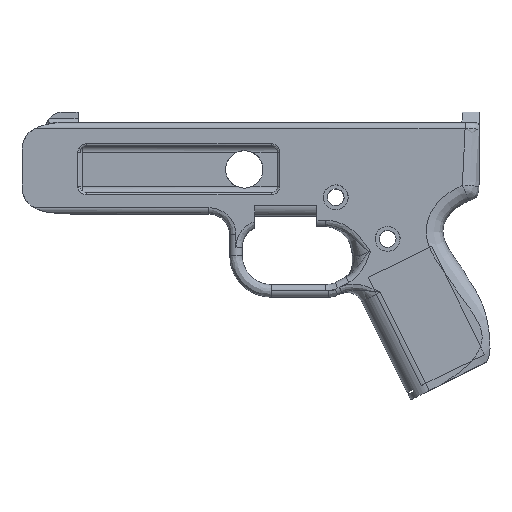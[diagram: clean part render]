
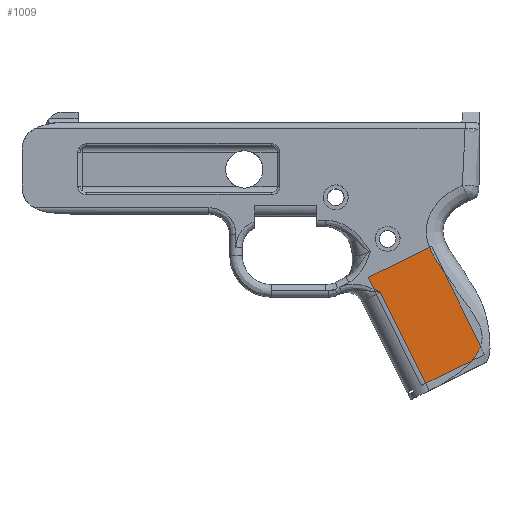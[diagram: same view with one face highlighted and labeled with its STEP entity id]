
A CAD part, top view. The second image highlights one B-rep face of the part: STEP entity #1009.
In plain terms, the highlighted planar face has unit normal (0, 0, 1).
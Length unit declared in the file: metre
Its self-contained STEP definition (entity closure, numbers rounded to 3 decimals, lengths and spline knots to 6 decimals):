
#1009=ADVANCED_FACE('0:4261',(#2004),#2005,.T.);
#2004=FACE_OUTER_BOUND('',#8349,.T.);
#2005=PLANE('',#8350);
#8349=EDGE_LOOP('',(#11330,#11331,#11332,#11333,#11334,#11335,#11336,#11337));
#8350=AXIS2_PLACEMENT_3D('',#11338,#11339,#11340);
#11330=ORIENTED_EDGE('',*,*,#12592,.T.);
#11331=ORIENTED_EDGE('',*,*,#12587,.F.);
#11332=ORIENTED_EDGE('',*,*,#12593,.T.);
#11333=ORIENTED_EDGE('',*,*,#12580,.F.);
#11334=ORIENTED_EDGE('',*,*,#12578,.F.);
#11335=ORIENTED_EDGE('',*,*,#12594,.T.);
#11336=ORIENTED_EDGE('',*,*,#12595,.T.);
#11337=ORIENTED_EDGE('',*,*,#12596,.T.);
#11338=CARTESIAN_POINT('',(0.072027,-0.137374,-0.119805));
#11339=DIRECTION('',(0.,0.,1.0));
#11340=DIRECTION('',(1.0,0.,0.0));
#12578=EDGE_CURVE('0:4321',#14399,#14389,#14401,.T.);
#12580=EDGE_CURVE('0:4324',#14389,#14403,#14404,.T.);
#12587=EDGE_CURVE('0:4342',#14413,#14415,#14416,.T.);
#12592=EDGE_CURVE('0:4351',#14421,#14415,#14422,.T.);
#12593=EDGE_CURVE('0:4354',#14413,#14403,#14423,.T.);
#12594=EDGE_CURVE('0:4357',#14399,#14424,#14425,.T.);
#12595=EDGE_CURVE('0:4360',#14424,#14426,#14427,.T.);
#12596=EDGE_CURVE('0:4363',#14426,#14421,#14428,.T.);
#14389=VERTEX_POINT('NONE',#23596);
#14399=VERTEX_POINT('NONE',#23615);
#14401=LINE('',#23626,#23627);
#14403=VERTEX_POINT('NONE',#23629);
#14404=LINE('',#23630,#23631);
#14413=VERTEX_POINT('NONE',#23646);
#14415=VERTEX_POINT('NONE',#23660);
#14416=LINE('',#23661,#23662);
#14421=VERTEX_POINT('NONE',#23674);
#14422=B_SPLINE_CURVE_WITH_KNOTS('',3,(#23675,#23676,#23677,#23678),.UNSPECIFIED.,.F.,.F.,(4,4),(0.0,1.0),.UNSPECIFIED.);
#14423=B_SPLINE_CURVE_WITH_KNOTS('',3,(#23679,#23680,#23681,#23682,#23683,#23684,#23685,#23686,#23687,#23688,#23689,#23690,#23691,#23692,#23693,#23694,#23695,#23696,#23697,#23698,#23699,#23700,#23701,#23702,#23703,#23704,#23705,#23706,#23707,#23708,#23709,#23710,#23711,#23712,#23713),.UNSPECIFIED.,.F.,.F.,(4,1,1,1,1,1,1,1,2,2,1,1,1,1,1,1,2,2,1,1,1,1,1,1,2,2,4),(0.0,0.125,0.1875,0.21875,0.234375,0.242188,0.246094,0.248047,0.249023,0.25,0.375,0.4375,0.46875,0.484375,0.492187,0.496094,0.498047,0.5,0.625,0.6875,0.71875,0.734375,0.742187,0.746094,0.748047,0.75,1.0),.UNSPECIFIED.);
#14424=VERTEX_POINT('NONE',#23714);
#14425=B_SPLINE_CURVE_WITH_KNOTS('',3,(#23715,#23716,#23717,#23718,#23719,#23720,#23721,#23722,#23723,#23724,#23725,#23726,#23727,#23728),.UNSPECIFIED.,.F.,.F.,(4,1,1,1,1,1,1,2,2,4),(0.0,0.25,0.375,0.4375,0.46875,0.484375,0.492188,0.496094,0.5,1.0),.UNSPECIFIED.);
#14426=VERTEX_POINT('NONE',#23729);
#14427=LINE('',#23730,#23731);
#14428=LINE('',#23732,#23733);
#23596=CARTESIAN_POINT('',(0.051871,-0.072504,-0.119805));
#23615=CARTESIAN_POINT('',(0.054708,-0.078321,-0.119805));
#23626=CARTESIAN_POINT('',(0.077297,-0.124634,-0.119805));
#23627=VECTOR('',#24437,1.0);
#23629=CARTESIAN_POINT('',(0.081371,-0.058116,-0.119805));
#23630=CARTESIAN_POINT('',(0.051871,-0.072504,-0.119805));
#23631=VECTOR('',#24438,1.0);
#23646=CARTESIAN_POINT('',(0.088584,-0.070218,-0.119805));
#23660=CARTESIAN_POINT('',(0.105946,-0.105814,-0.119805));
#23661=CARTESIAN_POINT('',(0.08243,-0.0576,-0.119805));
#23662=VECTOR('',#24442,1.0);
#23674=CARTESIAN_POINT('',(0.101572,-0.112794,-0.119805));
#23675=CARTESIAN_POINT('',(0.101572,-0.112794,-0.119805));
#23676=CARTESIAN_POINT('',(0.103685,-0.110425,-0.119805));
#23677=CARTESIAN_POINT('',(0.105143,-0.108098,-0.119805));
#23678=CARTESIAN_POINT('',(0.105946,-0.105814,-0.119805));
#23679=CARTESIAN_POINT('',(0.088584,-0.070218,-0.119805));
#23680=CARTESIAN_POINT('',(0.088139,-0.069591,-0.119805));
#23681=CARTESIAN_POINT('',(0.087551,-0.068761,-0.119805));
#23682=CARTESIAN_POINT('',(0.087005,-0.067981,-0.119805));
#23683=CARTESIAN_POINT('',(0.086767,-0.067639,-0.119805));
#23684=CARTESIAN_POINT('',(0.086656,-0.06748,-0.119805));
#23685=CARTESIAN_POINT('',(0.086603,-0.067403,-0.119805));
#23686=CARTESIAN_POINT('',(0.086578,-0.067366,-0.119805));
#23687=CARTESIAN_POINT('',(0.086565,-0.067347,-0.119805));
#23688=CARTESIAN_POINT('',(0.086559,-0.067339,-0.119805));
#23689=CARTESIAN_POINT('',(0.086556,-0.067334,-0.119805));
#23690=CARTESIAN_POINT('',(0.086555,-0.067333,-0.119805));
#23691=CARTESIAN_POINT('',(0.086182,-0.066791,-0.119805));
#23692=CARTESIAN_POINT('',(0.085662,-0.06602,-0.119805));
#23693=CARTESIAN_POINT('',(0.085115,-0.065181,-0.119805));
#23694=CARTESIAN_POINT('',(0.084856,-0.064776,-0.119805));
#23695=CARTESIAN_POINT('',(0.084731,-0.064577,-0.119805));
#23696=CARTESIAN_POINT('',(0.084669,-0.064479,-0.119805));
#23697=CARTESIAN_POINT('',(0.084638,-0.06443,-0.119805));
#23698=CARTESIAN_POINT('',(0.084625,-0.064409,-0.119805));
#23699=CARTESIAN_POINT('',(0.084617,-0.064395,-0.119805));
#23700=CARTESIAN_POINT('',(0.084613,-0.06439,-0.119805));
#23701=CARTESIAN_POINT('',(0.084272,-0.063844,-0.119805));
#23702=CARTESIAN_POINT('',(0.083799,-0.063058,-0.119805));
#23703=CARTESIAN_POINT('',(0.083303,-0.06218,-0.119805));
#23704=CARTESIAN_POINT('',(0.083069,-0.061751,-0.119805));
#23705=CARTESIAN_POINT('',(0.082955,-0.061539,-0.119805));
#23706=CARTESIAN_POINT('',(0.082899,-0.061433,-0.119805));
#23707=CARTESIAN_POINT('',(0.082871,-0.06138,-0.119805));
#23708=CARTESIAN_POINT('',(0.08286,-0.061358,-0.119805));
#23709=CARTESIAN_POINT('',(0.082852,-0.061343,-0.119805));
#23710=CARTESIAN_POINT('',(0.082848,-0.061336,-0.119805));
#23711=CARTESIAN_POINT('',(0.082267,-0.060228,-0.119805));
#23712=CARTESIAN_POINT('',(0.081776,-0.059158,-0.119805));
#23713=CARTESIAN_POINT('',(0.081371,-0.058116,-0.119805));
#23714=CARTESIAN_POINT('',(0.057717,-0.079683,-0.119805));
#23715=CARTESIAN_POINT('',(0.054708,-0.078321,-0.119805));
#23716=CARTESIAN_POINT('',(0.054933,-0.078418,-0.119805));
#23717=CARTESIAN_POINT('',(0.05529,-0.078575,-0.119805));
#23718=CARTESIAN_POINT('',(0.055743,-0.078778,-0.119805));
#23719=CARTESIAN_POINT('',(0.055978,-0.078884,-0.119805));
#23720=CARTESIAN_POINT('',(0.056097,-0.078938,-0.119805));
#23721=CARTESIAN_POINT('',(0.056158,-0.078966,-0.119805));
#23722=CARTESIAN_POINT('',(0.056188,-0.078979,-0.119805));
#23723=CARTESIAN_POINT('',(0.056201,-0.078985,-0.119805));
#23724=CARTESIAN_POINT('',(0.05621,-0.078989,-0.119805));
#23725=CARTESIAN_POINT('',(0.056216,-0.078992,-0.119805));
#23726=CARTESIAN_POINT('',(0.056552,-0.079145,-0.119805));
#23727=CARTESIAN_POINT('',(0.057051,-0.079375,-0.119805));
#23728=CARTESIAN_POINT('',(0.057717,-0.079683,-0.119805));
#23729=CARTESIAN_POINT('',(0.079624,-0.123499,-0.119805));
#23730=CARTESIAN_POINT('',(0.057717,-0.079683,-0.119805));
#23731=VECTOR('',#24444,1.0);
#23732=CARTESIAN_POINT('',(0.079624,-0.123499,-0.119805));
#23733=VECTOR('',#24445,1.0);
#24437=DIRECTION('',(-0.438,0.899,0.));
#24438=DIRECTION('',(0.899,0.438,0.));
#24442=DIRECTION('',(0.438,-0.899,0.));
#24444=DIRECTION('',(0.447,-0.894,0.));
#24445=DIRECTION('',(0.899,0.438,0.));
